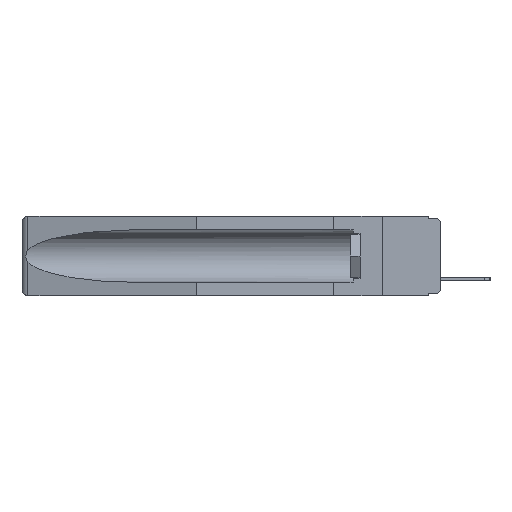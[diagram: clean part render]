
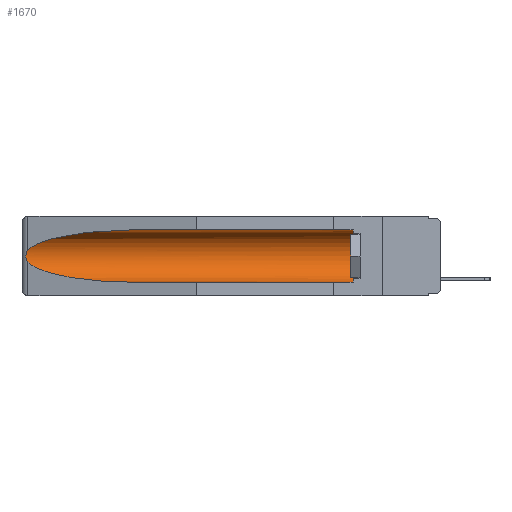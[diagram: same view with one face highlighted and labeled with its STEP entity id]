
A CAD part, left-side view. The second image highlights one B-rep face of the part: STEP entity #1670.
In plain terms, the highlighted cylindrical face has radius 2.857 mm (diameter 5.715 mm), a partial arc.
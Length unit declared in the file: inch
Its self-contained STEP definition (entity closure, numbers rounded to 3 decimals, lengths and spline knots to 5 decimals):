
#19 = CARTESIAN_POINT ( 'NONE',  ( 0.155, -0.30754, -0.059 ) ) ;
#134 = ORIENTED_EDGE ( 'NONE', *, *, #18167, .T. ) ;
#854 = CARTESIAN_POINT ( 'NONE',  ( 0.155, 0.126, -0.284 ) ) ;
#1136 = CARTESIAN_POINT ( 'NONE',  ( 0.2675, 1.53308, -0.17534 ) ) ;
#1239 = DIRECTION ( 'NONE',  ( 0., 1., 0. ) ) ;
#1670 = ADVANCED_FACE ( 'NONE', ( #3645 ), #11241, .F. ) ;
#1683 = CARTESIAN_POINT ( 'NONE',  ( 0.26597, 1.52961, -0.15275 ) ) ;
#1785 = CARTESIAN_POINT ( 'NONE',  ( 0.26537, 1.52718, -0.14972 ) ) ;
#1794 = DIRECTION ( 'NONE',  ( 0., 1., 0. ) ) ;
#1991 = DIRECTION ( 'NONE',  ( 0., 1., 0. ) ) ;
#2145 = CARTESIAN_POINT ( 'NONE',  ( 0.155, 0.126, -0.059 ) ) ;
#2528 = CARTESIAN_POINT ( 'NONE',  ( 0.26597, 1.5296, -0.19026 ) ) ;
#2989 = LINE ( 'NONE', #14046, #5723 ) ;
#3541 = CARTESIAN_POINT ( 'NONE',  ( 0.26537, 1.52718, -0.14972 ) ) ;
#3593 = CARTESIAN_POINT ( 'NONE',  ( 0.155, 1.07973, -0.284 ) ) ;
#3645 = FACE_OUTER_BOUND ( 'NONE', #11462, .T. ) ;
#3910 = B_SPLINE_CURVE_WITH_KNOTS ( 'NONE', 3,
 ( #3541, #1683, #23234, #4150, #19174, #1136, #18125, #8007, #2528, #21155 ),
 .UNSPECIFIED., .F., .F.,
 ( 4, 2, 2, 2, 4 ),
 ( 0., 0.00029, 0.00058, 0.00087, 0.00117 ),
 .UNSPECIFIED. ) ;
#4150 = CARTESIAN_POINT ( 'NONE',  ( 0.2673, 1.5327, -0.16383 ) ) ;
#5723 = VECTOR ( 'NONE', #1239, 39.37008 ) ;
#6355 = CARTESIAN_POINT ( 'NONE',  ( 0.155, 1.07973, -0.059 ) ) ;
#7000 = VERTEX_POINT ( 'NONE', #22252 ) ;
#7314 = CARTESIAN_POINT ( 'NONE',  ( 0.21114, 1.30732, -0.284 ) ) ;
#7508 = DIRECTION ( 'NONE',  ( 0., 0., 1. ) ) ;
#7705 = VERTEX_POINT ( 'NONE', #854 ) ;
#7853 = CARTESIAN_POINT ( 'NONE',  ( 0.26537, 1.52718, -0.19328 ) ) ;
#8007 = CARTESIAN_POINT ( 'NONE',  ( 0.26655, 1.53094, -0.18657 ) ) ;
#8350 = VERTEX_POINT ( 'NONE', #22862 ) ;
#9041 = VERTEX_POINT ( 'NONE', #7853 ) ;
#9153 =( BOUNDED_CURVE ( )  B_SPLINE_CURVE ( 3, ( #13207, #20770, #18903, #1785 ),
 .UNSPECIFIED., .F., .F. ) 
 B_SPLINE_CURVE_WITH_KNOTS ( ( 4, 4 ),
 ( 4.71239, 6.08839 ),
 .UNSPECIFIED. ) 
 CURVE ( )  GEOMETRIC_REPRESENTATION_ITEM ( )  RATIONAL_B_SPLINE_CURVE ( ( 1., 0.848, 0.848, 1. ) ) 
 REPRESENTATION_ITEM ( '' )  );
#10504 = VERTEX_POINT ( 'NONE', #6355 ) ;
#10608 = ORIENTED_EDGE ( 'NONE', *, *, #15072, .T. ) ;
#10727 =( BOUNDED_CURVE ( )  B_SPLINE_CURVE ( 3, ( #13867, #16763, #7314, #3593 ),
 .UNSPECIFIED., .F., .F. ) 
 B_SPLINE_CURVE_WITH_KNOTS ( ( 4, 4 ),
 ( 0.1948, 1.5708 ),
 .UNSPECIFIED. ) 
 CURVE ( )  GEOMETRIC_REPRESENTATION_ITEM ( )  RATIONAL_B_SPLINE_CURVE ( ( 1., 0.848, 0.848, 1. ) ) 
 REPRESENTATION_ITEM ( '' )  );
#11113 = EDGE_CURVE ( 'NONE', #7705, #8350, #2989, .T. ) ;
#11241 = CYLINDRICAL_SURFACE ( 'NONE', #20551, 0.1125 ) ;
#11462 = EDGE_LOOP ( 'NONE', ( #14323, #10608, #22536, #19393, #134, #22343 ) ) ;
#12556 = EDGE_CURVE ( 'NONE', #24119, #10504, #18870, .T. ) ;
#12688 = CIRCLE ( 'NONE', #18629, 0.1125 ) ;
#12880 = CARTESIAN_POINT ( 'NONE',  ( 0.155, 0.126, -0.1715 ) ) ;
#13207 = CARTESIAN_POINT ( 'NONE',  ( 0.155, 1.07973, -0.059 ) ) ;
#13867 = CARTESIAN_POINT ( 'NONE',  ( 0.26537, 1.52718, -0.19328 ) ) ;
#14046 = CARTESIAN_POINT ( 'NONE',  ( 0.155, -0.30754, -0.284 ) ) ;
#14323 = ORIENTED_EDGE ( 'NONE', *, *, #24082, .T. ) ;
#15072 = EDGE_CURVE ( 'NONE', #7000, #9041, #3910, .T. ) ;
#16605 = DIRECTION ( 'NONE',  ( 0., -1., 0. ) ) ;
#16763 = CARTESIAN_POINT ( 'NONE',  ( 0.25451, 1.48313, -0.24835 ) ) ;
#16884 = VECTOR ( 'NONE', #1991, 39.37008 ) ;
#18125 = CARTESIAN_POINT ( 'NONE',  ( 0.2673, 1.53269, -0.17917 ) ) ;
#18167 = EDGE_CURVE ( 'NONE', #7705, #24119, #12688, .T. ) ;
#18629 = AXIS2_PLACEMENT_3D ( 'NONE', #12880, #16605, #24270 ) ;
#18792 = CARTESIAN_POINT ( 'NONE',  ( 0.155, -0.30754, -0.1715 ) ) ;
#18870 = LINE ( 'NONE', #19, #16884 ) ;
#18903 = CARTESIAN_POINT ( 'NONE',  ( 0.25451, 1.48313, -0.09465 ) ) ;
#19174 = CARTESIAN_POINT ( 'NONE',  ( 0.2675, 1.53308, -0.16763 ) ) ;
#19393 = ORIENTED_EDGE ( 'NONE', *, *, #11113, .F. ) ;
#19739 = EDGE_CURVE ( 'NONE', #9041, #8350, #10727, .T. ) ;
#20551 = AXIS2_PLACEMENT_3D ( 'NONE', #18792, #1794, #7508 ) ;
#20770 = CARTESIAN_POINT ( 'NONE',  ( 0.21114, 1.30732, -0.059 ) ) ;
#21155 = CARTESIAN_POINT ( 'NONE',  ( 0.26537, 1.52718, -0.19328 ) ) ;
#22252 = CARTESIAN_POINT ( 'NONE',  ( 0.26537, 1.52718, -0.14972 ) ) ;
#22343 = ORIENTED_EDGE ( 'NONE', *, *, #12556, .T. ) ;
#22536 = ORIENTED_EDGE ( 'NONE', *, *, #19739, .T. ) ;
#22862 = CARTESIAN_POINT ( 'NONE',  ( 0.155, 1.07973, -0.284 ) ) ;
#23234 = CARTESIAN_POINT ( 'NONE',  ( 0.26654, 1.53092, -0.15636 ) ) ;
#24082 = EDGE_CURVE ( 'NONE', #10504, #7000, #9153, .T. ) ;
#24119 = VERTEX_POINT ( 'NONE', #2145 ) ;
#24270 = DIRECTION ( 'NONE',  ( 0., 0., 1. ) ) ;
